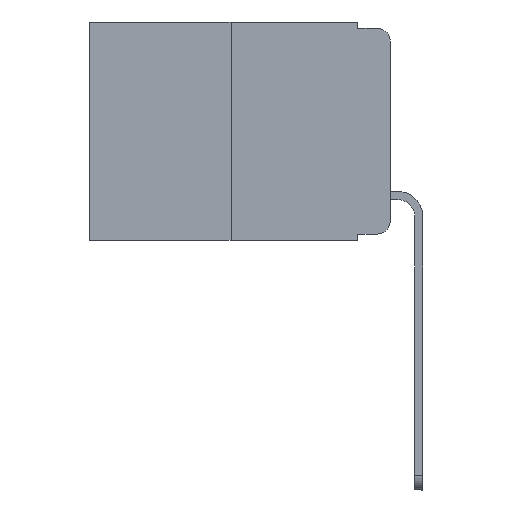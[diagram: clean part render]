
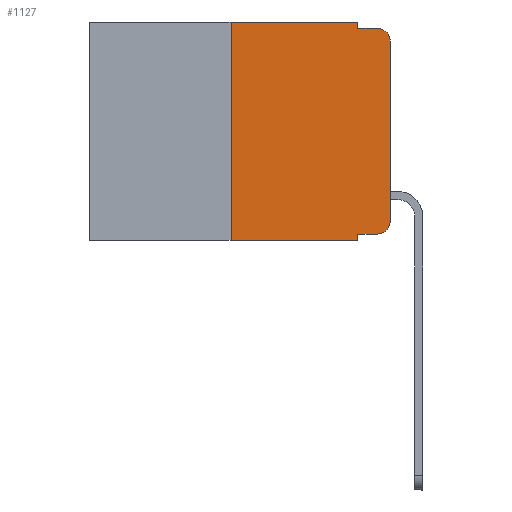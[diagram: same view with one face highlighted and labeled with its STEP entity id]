
A CAD part, left-side view. The second image highlights one B-rep face of the part: STEP entity #1127.
In plain terms, the highlighted planar face has unit normal (-1, 0, 0).
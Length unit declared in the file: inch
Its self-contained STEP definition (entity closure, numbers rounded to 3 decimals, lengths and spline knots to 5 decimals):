
#356 = VERTEX_POINT ( 'NONE', #15013 ) ;
#375 = CIRCLE ( 'NONE', #10108, 0.02 ) ;
#866 = LINE ( 'NONE', #17320, #11620 ) ;
#1127 = ADVANCED_FACE ( 'NONE', ( #3964 ), #13504, .F. ) ;
#1202 = LINE ( 'NONE', #14697, #9673 ) ;
#1264 = ORIENTED_EDGE ( 'NONE', *, *, #10022, .T. ) ;
#1273 = ORIENTED_EDGE ( 'NONE', *, *, #7028, .T. ) ;
#1351 = EDGE_CURVE ( 'NONE', #13669, #10975, #8762, .T. ) ;
#2272 = DIRECTION ( 'NONE',  ( 1., 0., 0. ) ) ;
#2292 = EDGE_CURVE ( 'NONE', #8992, #6356, #3453, .T. ) ;
#2992 = CARTESIAN_POINT ( 'NONE',  ( 0., 0.02, -0.333 ) ) ;
#3139 = DIRECTION ( 'NONE',  ( 0., 0., -1. ) ) ;
#3453 = LINE ( 'NONE', #13181, #14568 ) ;
#3964 = FACE_OUTER_BOUND ( 'NONE', #15931, .T. ) ;
#4009 = DIRECTION ( 'NONE',  ( 0., -1., 0. ) ) ;
#4093 = CARTESIAN_POINT ( 'NONE',  ( 0., 0., 0. ) ) ;
#4384 = ORIENTED_EDGE ( 'NONE', *, *, #7388, .F. ) ;
#4680 = VERTEX_POINT ( 'NONE', #2992 ) ;
#5324 = ORIENTED_EDGE ( 'NONE', *, *, #10266, .F. ) ;
#5963 = DIRECTION ( 'NONE',  ( 0., -1., 0. ) ) ;
#6154 = ORIENTED_EDGE ( 'NONE', *, *, #2292, .F. ) ;
#6356 = VERTEX_POINT ( 'NONE', #16670 ) ;
#6625 = VERTEX_POINT ( 'NONE', #17551 ) ;
#7028 = EDGE_CURVE ( 'NONE', #12292, #13669, #8058, .T. ) ;
#7060 = EDGE_CURVE ( 'NONE', #4680, #12292, #375, .T. ) ;
#7264 = VERTEX_POINT ( 'NONE', #12441 ) ;
#7388 = EDGE_CURVE ( 'NONE', #6625, #10616, #866, .T. ) ;
#7472 = EDGE_CURVE ( 'NONE', #356, #10975, #1202, .T. ) ;
#7696 = CARTESIAN_POINT ( 'NONE',  ( 0., 0., -0.03 ) ) ;
#7780 = DIRECTION ( 'NONE',  ( 0., -1., 0. ) ) ;
#7816 = CARTESIAN_POINT ( 'NONE',  ( 0., 0.02, -0.01 ) ) ;
#8058 = LINE ( 'NONE', #4093, #12661 ) ;
#8101 = CARTESIAN_POINT ( 'NONE',  ( 0., 0.051, 0. ) ) ;
#8470 = CARTESIAN_POINT ( 'NONE',  ( 0., 0.051, -0.333 ) ) ;
#8608 = DIRECTION ( 'NONE',  ( 0., 0., 1. ) ) ;
#8762 = CIRCLE ( 'NONE', #10193, 0.02 ) ;
#8992 = VERTEX_POINT ( 'NONE', #8470 ) ;
#9053 = CARTESIAN_POINT ( 'NONE',  ( 0., 0.473, -0.343 ) ) ;
#9673 = VECTOR ( 'NONE', #7780, 39.37008 ) ;
#9846 = LINE ( 'NONE', #12549, #10664 ) ;
#9865 = EDGE_CURVE ( 'NONE', #7264, #6625, #9846, .T. ) ;
#10022 = EDGE_CURVE ( 'NONE', #7264, #6356, #17163, .T. ) ;
#10108 = AXIS2_PLACEMENT_3D ( 'NONE', #12266, #16414, #10656 ) ;
#10158 = CARTESIAN_POINT ( 'NONE',  ( 0., 0.02, -0.03 ) ) ;
#10193 = AXIS2_PLACEMENT_3D ( 'NONE', #10158, #15572, #3139 ) ;
#10266 = EDGE_CURVE ( 'NONE', #10616, #356, #11002, .T. ) ;
#10616 = VERTEX_POINT ( 'NONE', #8101 ) ;
#10619 = CARTESIAN_POINT ( 'NONE',  ( 0., 0.473, 0. ) ) ;
#10656 = DIRECTION ( 'NONE',  ( 0., 0., -1. ) ) ;
#10664 = VECTOR ( 'NONE', #8608, 39.37008 ) ;
#10843 = CARTESIAN_POINT ( 'NONE',  ( 0., 0.051, -0.333 ) ) ;
#10957 = ORIENTED_EDGE ( 'NONE', *, *, #7472, .F. ) ;
#10975 = VERTEX_POINT ( 'NONE', #7816 ) ;
#11002 = LINE ( 'NONE', #12347, #17311 ) ;
#11620 = VECTOR ( 'NONE', #5963, 39.37008 ) ;
#11790 = ORIENTED_EDGE ( 'NONE', *, *, #1351, .T. ) ;
#12266 = CARTESIAN_POINT ( 'NONE',  ( 0., 0.02, -0.313 ) ) ;
#12292 = VERTEX_POINT ( 'NONE', #12355 ) ;
#12347 = CARTESIAN_POINT ( 'NONE',  ( 0., 0.051, 0. ) ) ;
#12355 = CARTESIAN_POINT ( 'NONE',  ( 0., 0., -0.313 ) ) ;
#12441 = CARTESIAN_POINT ( 'NONE',  ( 0., 0.25, -0.343 ) ) ;
#12524 = ORIENTED_EDGE ( 'NONE', *, *, #9865, .F. ) ;
#12549 = CARTESIAN_POINT ( 'NONE',  ( 0., 0.25, 0. ) ) ;
#12661 = VECTOR ( 'NONE', #14810, 39.37008 ) ;
#13181 = CARTESIAN_POINT ( 'NONE',  ( 0., 0.051, 0. ) ) ;
#13272 = DIRECTION ( 'NONE',  ( 0., -1., 0. ) ) ;
#13419 = ORIENTED_EDGE ( 'NONE', *, *, #7060, .T. ) ;
#13504 = PLANE ( 'NONE',  #13608 ) ;
#13608 = AXIS2_PLACEMENT_3D ( 'NONE', #10619, #2272, #16289 ) ;
#13669 = VERTEX_POINT ( 'NONE', #7696 ) ;
#14483 = VECTOR ( 'NONE', #13272, 39.37008 ) ;
#14568 = VECTOR ( 'NONE', #17413, 39.37008 ) ;
#14697 = CARTESIAN_POINT ( 'NONE',  ( 0., 0.051, -0.01 ) ) ;
#14699 = EDGE_CURVE ( 'NONE', #8992, #4680, #16246, .T. ) ;
#14810 = DIRECTION ( 'NONE',  ( 0., 0., 1. ) ) ;
#15013 = CARTESIAN_POINT ( 'NONE',  ( 0., 0.051, -0.01 ) ) ;
#15117 = VECTOR ( 'NONE', #4009, 39.37008 ) ;
#15572 = DIRECTION ( 'NONE',  ( -1., 0., 0. ) ) ;
#15931 = EDGE_LOOP ( 'NONE', ( #1273, #11790, #10957, #5324, #4384, #12524, #1264, #6154, #16162, #13419 ) ) ;
#16162 = ORIENTED_EDGE ( 'NONE', *, *, #14699, .T. ) ;
#16246 = LINE ( 'NONE', #10843, #15117 ) ;
#16289 = DIRECTION ( 'NONE',  ( 0., 0., -1. ) ) ;
#16414 = DIRECTION ( 'NONE',  ( -1., 0., 0. ) ) ;
#16499 = DIRECTION ( 'NONE',  ( 0., 0., -1. ) ) ;
#16670 = CARTESIAN_POINT ( 'NONE',  ( 0., 0.051, -0.343 ) ) ;
#17163 = LINE ( 'NONE', #9053, #14483 ) ;
#17311 = VECTOR ( 'NONE', #16499, 39.37008 ) ;
#17320 = CARTESIAN_POINT ( 'NONE',  ( 0., 0.473, 0. ) ) ;
#17413 = DIRECTION ( 'NONE',  ( 0., 0., -1. ) ) ;
#17551 = CARTESIAN_POINT ( 'NONE',  ( 0., 0.25, 0. ) ) ;
